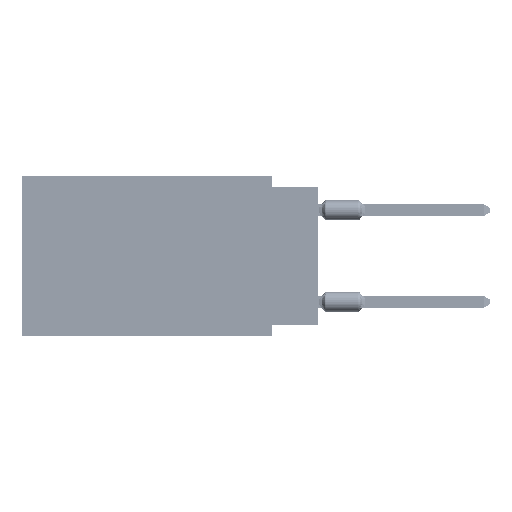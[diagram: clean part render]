
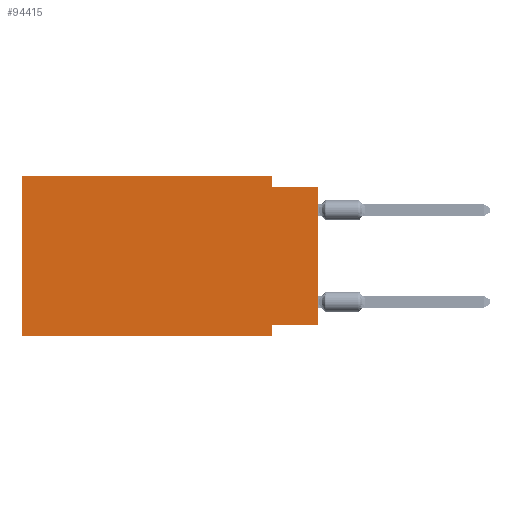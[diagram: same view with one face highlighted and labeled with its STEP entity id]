
A CAD part, left-side view. The second image highlights one B-rep face of the part: STEP entity #94415.
In plain terms, the highlighted planar face has unit normal (-1, 0, 0).
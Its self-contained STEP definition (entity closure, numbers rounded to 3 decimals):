
#187 = CARTESIAN_POINT ( 'NONE',  ( 0., 2.54, -8.89 ) ) ;
#1768 = DIRECTION ( 'NONE',  ( 0., -1., 0. ) ) ;
#3821 = LINE ( 'NONE', #63210, #67885 ) ;
#4733 = VERTEX_POINT ( 'NONE', #44620 ) ;
#11363 = EDGE_CURVE ( 'NONE', #49462, #12161, #55764, .T. ) ;
#12161 = VERTEX_POINT ( 'NONE', #18133 ) ;
#13405 = CARTESIAN_POINT ( 'NONE',  ( 0., 0., -0.635 ) ) ;
#15109 = VERTEX_POINT ( 'NONE', #187 ) ;
#15670 = CARTESIAN_POINT ( 'NONE',  ( 0., 16.383, -8.89 ) ) ;
#15877 = PLANE ( 'NONE',  #74385 ) ;
#16390 = VERTEX_POINT ( 'NONE', #15670 ) ;
#16856 = CARTESIAN_POINT ( 'NONE',  ( 0., 16.383, 0. ) ) ;
#18133 = CARTESIAN_POINT ( 'NONE',  ( 0., 2.54, -0.635 ) ) ;
#19462 = VECTOR ( 'NONE', #68061, 1000. ) ;
#22727 = DIRECTION ( 'NONE',  ( 0., -1., 0. ) ) ;
#23104 = CARTESIAN_POINT ( 'NONE',  ( 0., 0., -8.255 ) ) ;
#23359 = FACE_OUTER_BOUND ( 'NONE', #26511, .T. ) ;
#23737 = CARTESIAN_POINT ( 'NONE',  ( 0., 16.383, -8.89 ) ) ;
#25910 = VECTOR ( 'NONE', #56255, 1000. ) ;
#26328 = CARTESIAN_POINT ( 'NONE',  ( 0., 2.54, 0. ) ) ;
#26511 = EDGE_LOOP ( 'NONE', ( #32993, #65112, #47113, #95330, #59240, #27736, #36823, #39102 ) ) ;
#27736 = ORIENTED_EDGE ( 'NONE', *, *, #77743, .T. ) ;
#32322 = DIRECTION ( 'NONE',  ( 0., 0., -1. ) ) ;
#32993 = ORIENTED_EDGE ( 'NONE', *, *, #81736, .T. ) ;
#35340 = CARTESIAN_POINT ( 'NONE',  ( 0., 2.54, -8.89 ) ) ;
#36823 = ORIENTED_EDGE ( 'NONE', *, *, #50523, .F. ) ;
#37658 = LINE ( 'NONE', #61597, #19462 ) ;
#38959 = CARTESIAN_POINT ( 'NONE',  ( 0., 2.54, 0. ) ) ;
#39093 = VECTOR ( 'NONE', #70213, 1000. ) ;
#39102 = ORIENTED_EDGE ( 'NONE', *, *, #82245, .F. ) ;
#41114 = CARTESIAN_POINT ( 'NONE',  ( 0., 2.54, -8.255 ) ) ;
#43602 = VECTOR ( 'NONE', #1768, 1000. ) ;
#44180 = EDGE_CURVE ( 'NONE', #78887, #49462, #68580, .T. ) ;
#44620 = CARTESIAN_POINT ( 'NONE',  ( 0., 0., -8.255 ) ) ;
#45530 = DIRECTION ( 'NONE',  ( 0., 1., 0. ) ) ;
#46163 = CARTESIAN_POINT ( 'NONE',  ( 0., 16.383, 0. ) ) ;
#47113 = ORIENTED_EDGE ( 'NONE', *, *, #11363, .F. ) ;
#47284 = DIRECTION ( 'NONE',  ( 1., 0., 0. ) ) ;
#49462 = VERTEX_POINT ( 'NONE', #38959 ) ;
#50523 = EDGE_CURVE ( 'NONE', #95021, #15109, #59747, .T. ) ;
#54799 = LINE ( 'NONE', #70720, #39093 ) ;
#55764 = LINE ( 'NONE', #26328, #25910 ) ;
#56255 = DIRECTION ( 'NONE',  ( 0., 0., -1. ) ) ;
#58666 = CARTESIAN_POINT ( 'NONE',  ( 0., 16.383, 0. ) ) ;
#59240 = ORIENTED_EDGE ( 'NONE', *, *, #82800, .F. ) ;
#59747 = LINE ( 'NONE', #35340, #64075 ) ;
#61597 = CARTESIAN_POINT ( 'NONE',  ( 0., 0., -0.635 ) ) ;
#63210 = CARTESIAN_POINT ( 'NONE',  ( 0., 16.383, 0. ) ) ;
#64075 = VECTOR ( 'NONE', #95636, 1000. ) ;
#65112 = ORIENTED_EDGE ( 'NONE', *, *, #91807, .F. ) ;
#67885 = VECTOR ( 'NONE', #71633, 1000. ) ;
#68061 = DIRECTION ( 'NONE',  ( 0., -1., 0. ) ) ;
#68580 = LINE ( 'NONE', #46163, #95220 ) ;
#70063 = LINE ( 'NONE', #23737, #43602 ) ;
#70213 = DIRECTION ( 'NONE',  ( 0., 0., 1. ) ) ;
#70720 = CARTESIAN_POINT ( 'NONE',  ( 0., 0., 0. ) ) ;
#71633 = DIRECTION ( 'NONE',  ( 0., 0., 1. ) ) ;
#74385 = AXIS2_PLACEMENT_3D ( 'NONE', #16856, #47284, #32322 ) ;
#75764 = VERTEX_POINT ( 'NONE', #13405 ) ;
#77743 = EDGE_CURVE ( 'NONE', #16390, #15109, #70063, .T. ) ;
#78887 = VERTEX_POINT ( 'NONE', #58666 ) ;
#81736 = EDGE_CURVE ( 'NONE', #4733, #75764, #54799, .T. ) ;
#82245 = EDGE_CURVE ( 'NONE', #4733, #95021, #83410, .T. ) ;
#82800 = EDGE_CURVE ( 'NONE', #16390, #78887, #3821, .T. ) ;
#83410 = LINE ( 'NONE', #23104, #98049 ) ;
#91807 = EDGE_CURVE ( 'NONE', #12161, #75764, #37658, .T. ) ;
#94415 = ADVANCED_FACE ( 'NONE', ( #23359 ), #15877, .F. ) ;
#95021 = VERTEX_POINT ( 'NONE', #41114 ) ;
#95220 = VECTOR ( 'NONE', #22727, 1000. ) ;
#95330 = ORIENTED_EDGE ( 'NONE', *, *, #44180, .F. ) ;
#95636 = DIRECTION ( 'NONE',  ( 0., 0., -1. ) ) ;
#98049 = VECTOR ( 'NONE', #45530, 1000. ) ;
